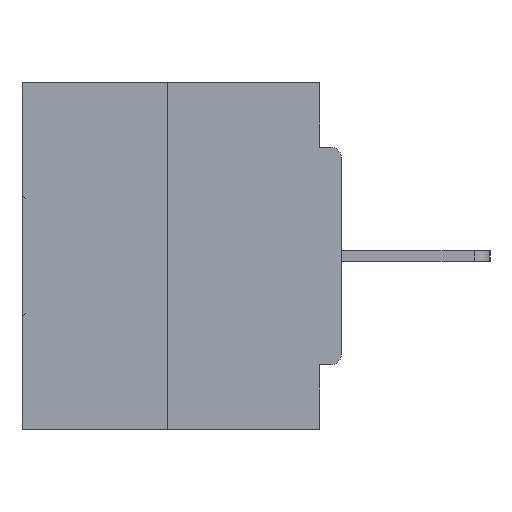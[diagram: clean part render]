
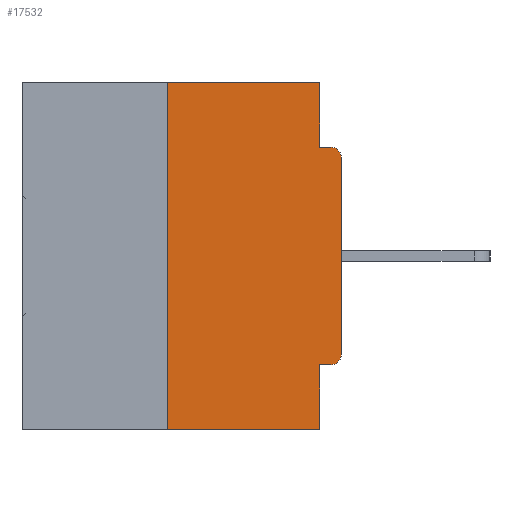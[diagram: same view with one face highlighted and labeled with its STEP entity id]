
A CAD part, left-side view. The second image highlights one B-rep face of the part: STEP entity #17532.
In plain terms, the highlighted planar face has unit normal (-1, 0, 0).
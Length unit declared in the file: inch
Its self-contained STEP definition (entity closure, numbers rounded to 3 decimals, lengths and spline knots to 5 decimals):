
#168 = VERTEX_POINT ( 'NONE', #36405 ) ;
#2630 = FACE_OUTER_BOUND ( 'NONE', #30119, .T. ) ;
#3354 = ORIENTED_EDGE ( 'NONE', *, *, #27760, .F. ) ;
#3607 = DIRECTION ( 'NONE',  ( 0., 0., -1. ) ) ;
#3858 = DIRECTION ( 'NONE',  ( 0., -1., 0. ) ) ;
#4091 = VERTEX_POINT ( 'NONE', #12666 ) ;
#4571 = VERTEX_POINT ( 'NONE', #19642 ) ;
#4922 = CARTESIAN_POINT ( 'NONE',  ( 0., 0.031, -0.0935 ) ) ;
#4953 = CARTESIAN_POINT ( 'NONE',  ( 0., 0.015, -0.0935 ) ) ;
#5709 = CARTESIAN_POINT ( 'NONE',  ( 0., 0.031, 0. ) ) ;
#5734 = VECTOR ( 'NONE', #17003, 39.37008 ) ;
#6111 = CARTESIAN_POINT ( 'NONE',  ( 0., 0.25, 0. ) ) ;
#6221 = EDGE_CURVE ( 'NONE', #37184, #9648, #11548, .T. ) ;
#6350 = EDGE_CURVE ( 'NONE', #4091, #9648, #27852, .T. ) ;
#6437 = CARTESIAN_POINT ( 'NONE',  ( 0., 0., -0.4065 ) ) ;
#6585 = VECTOR ( 'NONE', #32720, 39.37008 ) ;
#7084 = EDGE_CURVE ( 'NONE', #23331, #21567, #11462, .T. ) ;
#7112 = CARTESIAN_POINT ( 'NONE',  ( 0., 0.46, -0.5 ) ) ;
#7221 = DIRECTION ( 'NONE',  ( -1., 0., 0. ) ) ;
#8030 = AXIS2_PLACEMENT_3D ( 'NONE', #31982, #19688, #8559 ) ;
#8260 = LINE ( 'NONE', #13999, #30424 ) ;
#8559 = DIRECTION ( 'NONE',  ( 0., 0., -1. ) ) ;
#8887 = LINE ( 'NONE', #32668, #9791 ) ;
#9091 = ORIENTED_EDGE ( 'NONE', *, *, #6350, .T. ) ;
#9243 = DIRECTION ( 'NONE',  ( 0., 0., -1. ) ) ;
#9254 = ORIENTED_EDGE ( 'NONE', *, *, #33828, .F. ) ;
#9315 = LINE ( 'NONE', #6437, #6585 ) ;
#9648 = VERTEX_POINT ( 'NONE', #16200 ) ;
#9791 = VECTOR ( 'NONE', #35544, 39.37008 ) ;
#9846 = ORIENTED_EDGE ( 'NONE', *, *, #6221, .F. ) ;
#10402 = CARTESIAN_POINT ( 'NONE',  ( 0., 0.031, 0. ) ) ;
#11282 = LINE ( 'NONE', #26445, #5734 ) ;
#11462 = LINE ( 'NONE', #5709, #18527 ) ;
#11548 = LINE ( 'NONE', #17481, #16658 ) ;
#11573 = CARTESIAN_POINT ( 'NONE',  ( 0., 0., 0. ) ) ;
#11657 = EDGE_CURVE ( 'NONE', #21567, #27716, #8260, .T. ) ;
#12001 = ORIENTED_EDGE ( 'NONE', *, *, #11657, .F. ) ;
#12624 = DIRECTION ( 'NONE',  ( -1., 0., 0. ) ) ;
#12666 = CARTESIAN_POINT ( 'NONE',  ( 0., 0.25, -0.5 ) ) ;
#13639 = EDGE_CURVE ( 'NONE', #31765, #27716, #24974, .T. ) ;
#13938 = EDGE_CURVE ( 'NONE', #168, #37184, #9315, .T. ) ;
#13999 = CARTESIAN_POINT ( 'NONE',  ( 0., 0., -0.0935 ) ) ;
#14385 = EDGE_CURVE ( 'NONE', #4571, #31765, #32479, .T. ) ;
#16200 = CARTESIAN_POINT ( 'NONE',  ( 0., 0.031, -0.5 ) ) ;
#16658 = VECTOR ( 'NONE', #9243, 39.37008 ) ;
#17003 = DIRECTION ( 'NONE',  ( 0., 0., 1. ) ) ;
#17122 = DIRECTION ( 'NONE',  ( 0., 0., 1. ) ) ;
#17291 = EDGE_CURVE ( 'NONE', #168, #4571, #25201, .T. ) ;
#17398 = CARTESIAN_POINT ( 'NONE',  ( 0., 0., -0.1085 ) ) ;
#17481 = CARTESIAN_POINT ( 'NONE',  ( 0., 0.031, -0.5 ) ) ;
#17532 = ADVANCED_FACE ( 'NONE', ( #2630 ), #28926, .F. ) ;
#17882 = ORIENTED_EDGE ( 'NONE', *, *, #14385, .T. ) ;
#18527 = VECTOR ( 'NONE', #29507, 39.37008 ) ;
#18699 = ORIENTED_EDGE ( 'NONE', *, *, #13938, .F. ) ;
#19024 = AXIS2_PLACEMENT_3D ( 'NONE', #26670, #12624, #3607 ) ;
#19642 = CARTESIAN_POINT ( 'NONE',  ( 0., 0., -0.3915 ) ) ;
#19688 = DIRECTION ( 'NONE',  ( 1., 0., 0. ) ) ;
#21567 = VERTEX_POINT ( 'NONE', #4922 ) ;
#23331 = VERTEX_POINT ( 'NONE', #10402 ) ;
#24974 = CIRCLE ( 'NONE', #32928, 0.015 ) ;
#25002 = VECTOR ( 'NONE', #17122, 39.37008 ) ;
#25083 = DIRECTION ( 'NONE',  ( 0., 0., -1. ) ) ;
#25201 = CIRCLE ( 'NONE', #19024, 0.015 ) ;
#25220 = VERTEX_POINT ( 'NONE', #6111 ) ;
#26445 = CARTESIAN_POINT ( 'NONE',  ( 0., 0.25, 0. ) ) ;
#26670 = CARTESIAN_POINT ( 'NONE',  ( 0., 0.015, -0.3915 ) ) ;
#27216 = CARTESIAN_POINT ( 'NONE',  ( 0., 0.015, -0.1085 ) ) ;
#27716 = VERTEX_POINT ( 'NONE', #4953 ) ;
#27760 = EDGE_CURVE ( 'NONE', #4091, #25220, #11282, .T. ) ;
#27852 = LINE ( 'NONE', #7112, #35081 ) ;
#28926 = PLANE ( 'NONE',  #8030 ) ;
#29507 = DIRECTION ( 'NONE',  ( 0., 0., -1. ) ) ;
#30119 = EDGE_LOOP ( 'NONE', ( #9254, #3354, #9091, #9846, #18699, #31899, #17882, #32893, #12001, #35729 ) ) ;
#30424 = VECTOR ( 'NONE', #31668, 39.37008 ) ;
#31668 = DIRECTION ( 'NONE',  ( 0., -1., 0. ) ) ;
#31765 = VERTEX_POINT ( 'NONE', #17398 ) ;
#31897 = CARTESIAN_POINT ( 'NONE',  ( 0., 0.031, -0.4065 ) ) ;
#31899 = ORIENTED_EDGE ( 'NONE', *, *, #17291, .T. ) ;
#31982 = CARTESIAN_POINT ( 'NONE',  ( 0., 0.46, 0. ) ) ;
#32479 = LINE ( 'NONE', #11573, #25002 ) ;
#32668 = CARTESIAN_POINT ( 'NONE',  ( 0., 0.46, 0. ) ) ;
#32720 = DIRECTION ( 'NONE',  ( 0., 1., 0. ) ) ;
#32893 = ORIENTED_EDGE ( 'NONE', *, *, #13639, .T. ) ;
#32928 = AXIS2_PLACEMENT_3D ( 'NONE', #27216, #7221, #25083 ) ;
#33828 = EDGE_CURVE ( 'NONE', #25220, #23331, #8887, .T. ) ;
#35081 = VECTOR ( 'NONE', #3858, 39.37008 ) ;
#35544 = DIRECTION ( 'NONE',  ( 0., -1., 0. ) ) ;
#35729 = ORIENTED_EDGE ( 'NONE', *, *, #7084, .F. ) ;
#36405 = CARTESIAN_POINT ( 'NONE',  ( 0., 0.015, -0.4065 ) ) ;
#37184 = VERTEX_POINT ( 'NONE', #31897 ) ;
